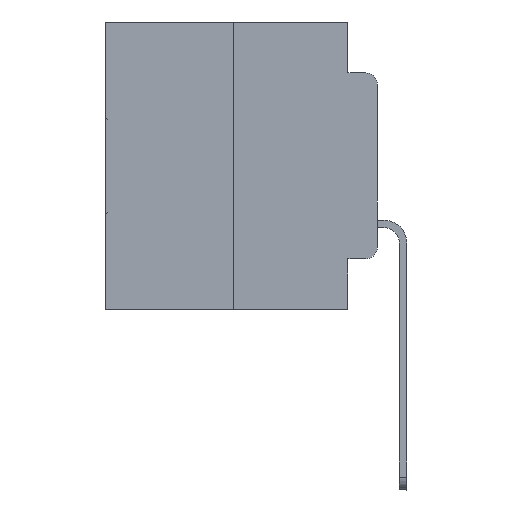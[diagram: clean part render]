
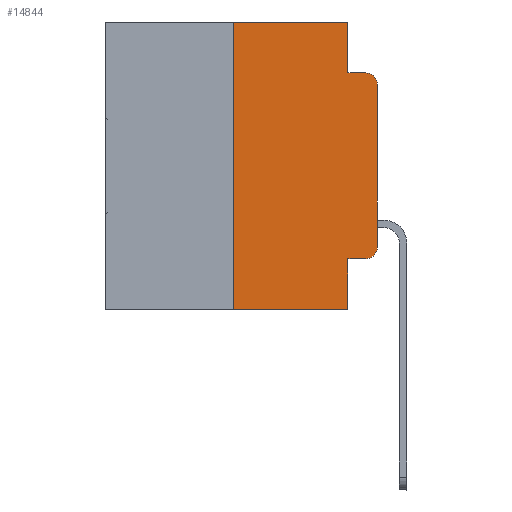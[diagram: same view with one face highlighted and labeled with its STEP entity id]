
A CAD part, left-side view. The second image highlights one B-rep face of the part: STEP entity #14844.
In plain terms, the highlighted planar face has unit normal (-1, 0, 0).
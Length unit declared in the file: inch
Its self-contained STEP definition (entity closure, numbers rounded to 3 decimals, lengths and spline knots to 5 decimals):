
#361 = VECTOR ( 'NONE', #17299, 39.37008 ) ;
#438 = EDGE_CURVE ( 'NONE', #5100, #22301, #18509, .T. ) ;
#686 = DIRECTION ( 'NONE',  ( 0., 0., -1. ) ) ;
#952 = CARTESIAN_POINT ( 'NONE',  ( 0., 0.051, -0.0885 ) ) ;
#1200 = VERTEX_POINT ( 'NONE', #11243 ) ;
#1341 = CARTESIAN_POINT ( 'NONE',  ( 0., 0.051, 0. ) ) ;
#1537 = EDGE_CURVE ( 'NONE', #5100, #16059, #21953, .T. ) ;
#1849 = VERTEX_POINT ( 'NONE', #24030 ) ;
#2269 = EDGE_CURVE ( 'NONE', #27864, #16059, #22850, .T. ) ;
#2526 = EDGE_CURVE ( 'NONE', #1200, #4659, #21748, .T. ) ;
#3101 = LINE ( 'NONE', #19438, #15062 ) ;
#3377 = VERTEX_POINT ( 'NONE', #7745 ) ;
#3618 = VECTOR ( 'NONE', #18536, 39.37008 ) ;
#4395 = ORIENTED_EDGE ( 'NONE', *, *, #2269, .T. ) ;
#4659 = VERTEX_POINT ( 'NONE', #14326 ) ;
#5086 = CARTESIAN_POINT ( 'NONE',  ( 0., 0.051, -0.4115 ) ) ;
#5100 = VERTEX_POINT ( 'NONE', #28399 ) ;
#5282 = VECTOR ( 'NONE', #686, 39.37008 ) ;
#6282 = DIRECTION ( 'NONE',  ( 0., 0., -1. ) ) ;
#6384 = EDGE_CURVE ( 'NONE', #3377, #13068, #15296, .T. ) ;
#6459 = ORIENTED_EDGE ( 'NONE', *, *, #438, .T. ) ;
#6592 = AXIS2_PLACEMENT_3D ( 'NONE', #7969, #17862, #6282 ) ;
#7031 = AXIS2_PLACEMENT_3D ( 'NONE', #17897, #24648, #29692 ) ;
#7333 = CIRCLE ( 'NONE', #15110, 0.02 ) ;
#7672 = ORIENTED_EDGE ( 'NONE', *, *, #2526, .F. ) ;
#7745 = CARTESIAN_POINT ( 'NONE',  ( 0., 0., -0.3915 ) ) ;
#7856 = ORIENTED_EDGE ( 'NONE', *, *, #18846, .F. ) ;
#7969 = CARTESIAN_POINT ( 'NONE',  ( 0., 0.473, 0. ) ) ;
#8007 = CIRCLE ( 'NONE', #7031, 0.02 ) ;
#8012 = DIRECTION ( 'NONE',  ( 0., 0., 1. ) ) ;
#8344 = DIRECTION ( 'NONE',  ( 0., -1., 0. ) ) ;
#8474 = VECTOR ( 'NONE', #21566, 39.37008 ) ;
#8840 = ORIENTED_EDGE ( 'NONE', *, *, #27845, .F. ) ;
#8882 = VERTEX_POINT ( 'NONE', #14716 ) ;
#8958 = EDGE_CURVE ( 'NONE', #13068, #4659, #7333, .T. ) ;
#9687 = CARTESIAN_POINT ( 'NONE',  ( 0., 0.473, 0. ) ) ;
#10019 = EDGE_LOOP ( 'NONE', ( #10448, #10838, #7672, #7856, #8840, #11173, #4395, #27416, #6459, #21436 ) ) ;
#10448 = ORIENTED_EDGE ( 'NONE', *, *, #6384, .T. ) ;
#10594 = DIRECTION ( 'NONE',  ( -1., 0., 0. ) ) ;
#10689 = PLANE ( 'NONE',  #6592 ) ;
#10838 = ORIENTED_EDGE ( 'NONE', *, *, #8958, .T. ) ;
#11173 = ORIENTED_EDGE ( 'NONE', *, *, #19935, .F. ) ;
#11243 = CARTESIAN_POINT ( 'NONE',  ( 0., 0.051, -0.0885 ) ) ;
#11537 = VECTOR ( 'NONE', #8012, 39.37008 ) ;
#12562 = CARTESIAN_POINT ( 'NONE',  ( 0., 0.02, -0.1085 ) ) ;
#12705 = CARTESIAN_POINT ( 'NONE',  ( 0., 0., 0. ) ) ;
#13068 = VERTEX_POINT ( 'NONE', #21093 ) ;
#13168 = DIRECTION ( 'NONE',  ( 0., 0., -1. ) ) ;
#14326 = CARTESIAN_POINT ( 'NONE',  ( 0., 0.02, -0.0885 ) ) ;
#14716 = CARTESIAN_POINT ( 'NONE',  ( 0., 0.051, 0. ) ) ;
#14844 = ADVANCED_FACE ( 'NONE', ( #17413 ), #10689, .F. ) ;
#15062 = VECTOR ( 'NONE', #26493, 39.37008 ) ;
#15110 = AXIS2_PLACEMENT_3D ( 'NONE', #12562, #10594, #13168 ) ;
#15296 = LINE ( 'NONE', #12705, #11537 ) ;
#16059 = VERTEX_POINT ( 'NONE', #22481 ) ;
#16389 = LINE ( 'NONE', #9687, #3618 ) ;
#17299 = DIRECTION ( 'NONE',  ( 0., -1., 0. ) ) ;
#17413 = FACE_OUTER_BOUND ( 'NONE', #10019, .T. ) ;
#17862 = DIRECTION ( 'NONE',  ( 1., 0., 0. ) ) ;
#17897 = CARTESIAN_POINT ( 'NONE',  ( 0., 0.02, -0.3915 ) ) ;
#18509 = LINE ( 'NONE', #5086, #8474 ) ;
#18536 = DIRECTION ( 'NONE',  ( 0., -1., 0. ) ) ;
#18846 = EDGE_CURVE ( 'NONE', #8882, #1200, #19991, .T. ) ;
#19438 = CARTESIAN_POINT ( 'NONE',  ( 0., 0.25, 0. ) ) ;
#19935 = EDGE_CURVE ( 'NONE', #27864, #1849, #3101, .T. ) ;
#19991 = LINE ( 'NONE', #1341, #29673 ) ;
#21093 = CARTESIAN_POINT ( 'NONE',  ( 0., 0., -0.1085 ) ) ;
#21436 = ORIENTED_EDGE ( 'NONE', *, *, #28017, .T. ) ;
#21566 = DIRECTION ( 'NONE',  ( 0., -1., 0. ) ) ;
#21748 = LINE ( 'NONE', #952, #361 ) ;
#21901 = CARTESIAN_POINT ( 'NONE',  ( 0., 0.25, -0.5 ) ) ;
#21953 = LINE ( 'NONE', #29546, #5282 ) ;
#22301 = VERTEX_POINT ( 'NONE', #27026 ) ;
#22481 = CARTESIAN_POINT ( 'NONE',  ( 0., 0.051, -0.5 ) ) ;
#22850 = LINE ( 'NONE', #25145, #24769 ) ;
#24030 = CARTESIAN_POINT ( 'NONE',  ( 0., 0.25, 0. ) ) ;
#24648 = DIRECTION ( 'NONE',  ( -1., 0., 0. ) ) ;
#24744 = DIRECTION ( 'NONE',  ( 0., 0., -1. ) ) ;
#24769 = VECTOR ( 'NONE', #8344, 39.37008 ) ;
#25145 = CARTESIAN_POINT ( 'NONE',  ( 0., 0.473, -0.5 ) ) ;
#26493 = DIRECTION ( 'NONE',  ( 0., 0., 1. ) ) ;
#27026 = CARTESIAN_POINT ( 'NONE',  ( 0., 0.02, -0.4115 ) ) ;
#27416 = ORIENTED_EDGE ( 'NONE', *, *, #1537, .F. ) ;
#27845 = EDGE_CURVE ( 'NONE', #1849, #8882, #16389, .T. ) ;
#27864 = VERTEX_POINT ( 'NONE', #21901 ) ;
#28017 = EDGE_CURVE ( 'NONE', #22301, #3377, #8007, .T. ) ;
#28399 = CARTESIAN_POINT ( 'NONE',  ( 0., 0.051, -0.4115 ) ) ;
#29546 = CARTESIAN_POINT ( 'NONE',  ( 0., 0.051, 0. ) ) ;
#29673 = VECTOR ( 'NONE', #24744, 39.37008 ) ;
#29692 = DIRECTION ( 'NONE',  ( 0., 0., -1. ) ) ;
